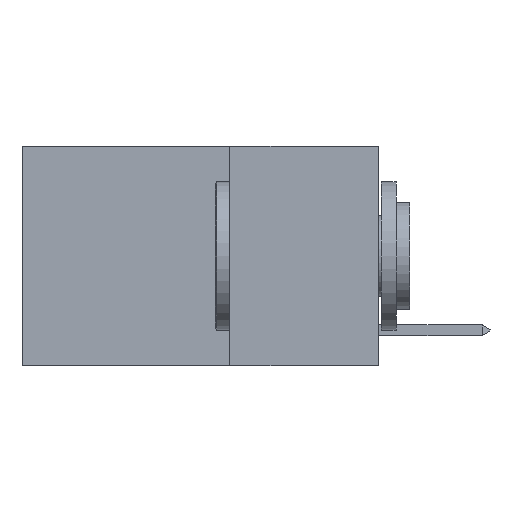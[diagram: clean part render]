
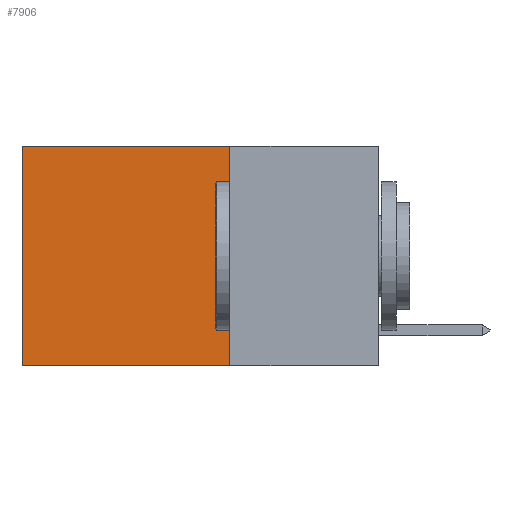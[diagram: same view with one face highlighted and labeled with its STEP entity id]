
A CAD part, left-side view. The second image highlights one B-rep face of the part: STEP entity #7906.
In plain terms, the highlighted planar face has unit normal (-1, 0, 0).
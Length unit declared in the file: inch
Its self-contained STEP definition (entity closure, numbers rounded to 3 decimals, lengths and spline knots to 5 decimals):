
#67 = VECTOR ( 'NONE', #8914, 39.37008 ) ;
#202 = VECTOR ( 'NONE', #2882, 39.37008 ) ;
#341 = VECTOR ( 'NONE', #11273, 39.37008 ) ;
#1294 = CARTESIAN_POINT ( 'NONE',  ( 0.2625, 0.25, -0.37 ) ) ;
#1666 = LINE ( 'NONE', #8315, #341 ) ;
#1775 = CARTESIAN_POINT ( 'NONE',  ( 0.2625, 0.6, -0.37 ) ) ;
#2038 = VERTEX_POINT ( 'NONE', #11623 ) ;
#2298 = ORIENTED_EDGE ( 'NONE', *, *, #8516, .F. ) ;
#2348 = ORIENTED_EDGE ( 'NONE', *, *, #10776, .F. ) ;
#2882 = DIRECTION ( 'NONE',  ( 0., 1., 0. ) ) ;
#3149 = ORIENTED_EDGE ( 'NONE', *, *, #7592, .T. ) ;
#3349 = CARTESIAN_POINT ( 'NONE',  ( 0.2625, 0.25, 0. ) ) ;
#3995 = LINE ( 'NONE', #1294, #4740 ) ;
#4027 = EDGE_LOOP ( 'NONE', ( #9786, #2298, #2348, #3149 ) ) ;
#4530 = AXIS2_PLACEMENT_3D ( 'NONE', #12081, #6493, #6254 ) ;
#4665 = PLANE ( 'NONE',  #4530 ) ;
#4740 = VECTOR ( 'NONE', #4806, 39.37008 ) ;
#4806 = DIRECTION ( 'NONE',  ( 0., 1., 0. ) ) ;
#4891 = CARTESIAN_POINT ( 'NONE',  ( 0.2625, 0.25, 0. ) ) ;
#5425 = EDGE_CURVE ( 'NONE', #11330, #9556, #1666, .T. ) ;
#6254 = DIRECTION ( 'NONE',  ( 0., 0., -1. ) ) ;
#6437 = FACE_OUTER_BOUND ( 'NONE', #4027, .T. ) ;
#6493 = DIRECTION ( 'NONE',  ( 1., 0., 0. ) ) ;
#7592 = EDGE_CURVE ( 'NONE', #2038, #11330, #10376, .T. ) ;
#7906 = ADVANCED_FACE ( 'NONE', ( #6437 ), #4665, .F. ) ;
#8315 = CARTESIAN_POINT ( 'NONE',  ( 0.2625, 0.6, 0. ) ) ;
#8516 = EDGE_CURVE ( 'NONE', #11149, #9556, #3995, .T. ) ;
#8914 = DIRECTION ( 'NONE',  ( 0., 0., -1. ) ) ;
#9556 = VERTEX_POINT ( 'NONE', #1775 ) ;
#9786 = ORIENTED_EDGE ( 'NONE', *, *, #5425, .T. ) ;
#10295 = CARTESIAN_POINT ( 'NONE',  ( 0.2625, 0.6, 0. ) ) ;
#10376 = LINE ( 'NONE', #4891, #202 ) ;
#10776 = EDGE_CURVE ( 'NONE', #2038, #11149, #11819, .T. ) ;
#10916 = CARTESIAN_POINT ( 'NONE',  ( 0.2625, 0.25, -0.37 ) ) ;
#11149 = VERTEX_POINT ( 'NONE', #10916 ) ;
#11273 = DIRECTION ( 'NONE',  ( 0., 0., -1. ) ) ;
#11330 = VERTEX_POINT ( 'NONE', #10295 ) ;
#11623 = CARTESIAN_POINT ( 'NONE',  ( 0.2625, 0.25, 0. ) ) ;
#11819 = LINE ( 'NONE', #3349, #67 ) ;
#12081 = CARTESIAN_POINT ( 'NONE',  ( 0.2625, 0.25, 0. ) ) ;
